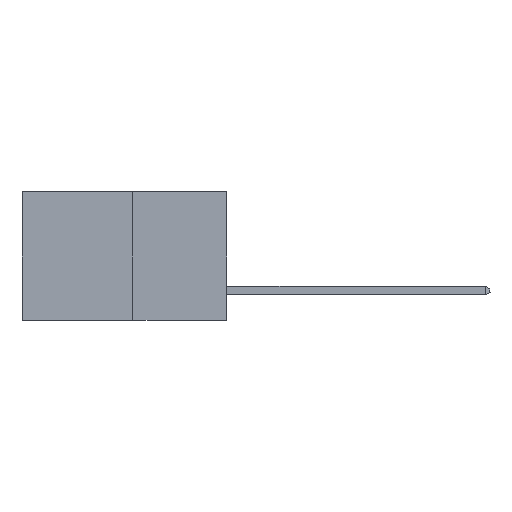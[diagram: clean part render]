
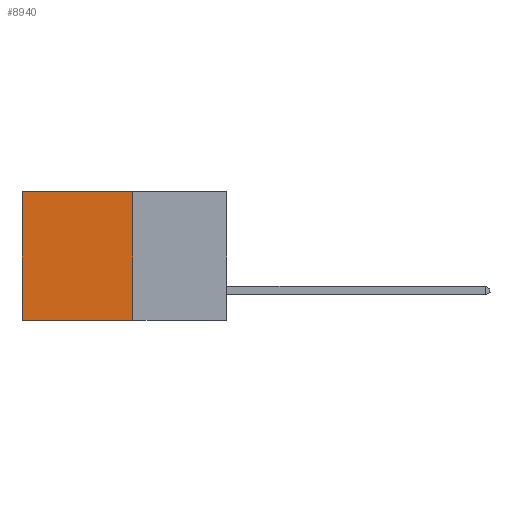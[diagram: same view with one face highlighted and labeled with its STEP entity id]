
A CAD part, left-side view. The second image highlights one B-rep face of the part: STEP entity #8940.
In plain terms, the highlighted planar face has unit normal (-1, 0, 0).
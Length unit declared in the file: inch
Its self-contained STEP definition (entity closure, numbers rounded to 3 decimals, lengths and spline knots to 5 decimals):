
#193 = DIRECTION ( 'NONE',  ( 0., 1., 0. ) ) ;
#296 = CARTESIAN_POINT ( 'NONE',  ( 0.277, 0.27, 0. ) ) ;
#1221 = CARTESIAN_POINT ( 'NONE',  ( 0.277, 0.59, -0.37 ) ) ;
#1253 = EDGE_CURVE ( 'NONE', #1837, #8691, #19390, .T. ) ;
#1837 = VERTEX_POINT ( 'NONE', #17313 ) ;
#3182 = DIRECTION ( 'NONE',  ( 0., 0., -1. ) ) ;
#3802 = ORIENTED_EDGE ( 'NONE', *, *, #19534, .F. ) ;
#5381 = CARTESIAN_POINT ( 'NONE',  ( 0.277, 0.27, -0.37 ) ) ;
#5723 = VECTOR ( 'NONE', #3182, 39.37008 ) ;
#6802 = EDGE_CURVE ( 'NONE', #17176, #8691, #8059, .T. ) ;
#8059 = LINE ( 'NONE', #17835, #20864 ) ;
#8691 = VERTEX_POINT ( 'NONE', #1221 ) ;
#8940 = ADVANCED_FACE ( 'NONE', ( #11349 ), #19799, .F. ) ;
#9045 = DIRECTION ( 'NONE',  ( 0., 0., -1. ) ) ;
#10345 = CARTESIAN_POINT ( 'NONE',  ( 0.277, 0.27, 0. ) ) ;
#10465 = EDGE_CURVE ( 'NONE', #12814, #1837, #13393, .T. ) ;
#10470 = VECTOR ( 'NONE', #9045, 39.37008 ) ;
#11349 = FACE_OUTER_BOUND ( 'NONE', #14837, .T. ) ;
#11478 = ORIENTED_EDGE ( 'NONE', *, *, #1253, .T. ) ;
#11710 = CARTESIAN_POINT ( 'NONE',  ( 0.277, 0.27, -0.37 ) ) ;
#12140 = CARTESIAN_POINT ( 'NONE',  ( 0.277, 0.59, -0.37 ) ) ;
#12814 = VERTEX_POINT ( 'NONE', #10345 ) ;
#12886 = VECTOR ( 'NONE', #193, 39.37008 ) ;
#13393 = LINE ( 'NONE', #296, #12886 ) ;
#14190 = ORIENTED_EDGE ( 'NONE', *, *, #6802, .F. ) ;
#14837 = EDGE_LOOP ( 'NONE', ( #11478, #14190, #3802, #16027 ) ) ;
#15682 = LINE ( 'NONE', #11710, #5723 ) ;
#16027 = ORIENTED_EDGE ( 'NONE', *, *, #10465, .T. ) ;
#17176 = VERTEX_POINT ( 'NONE', #5381 ) ;
#17313 = CARTESIAN_POINT ( 'NONE',  ( 0.277, 0.59, 0. ) ) ;
#17813 = DIRECTION ( 'NONE',  ( 0., 1., 0. ) ) ;
#17835 = CARTESIAN_POINT ( 'NONE',  ( 0.277, 0.27, -0.37 ) ) ;
#19374 = AXIS2_PLACEMENT_3D ( 'NONE', #19778, #19772, #19723 ) ;
#19390 = LINE ( 'NONE', #12140, #10470 ) ;
#19534 = EDGE_CURVE ( 'NONE', #12814, #17176, #15682, .T. ) ;
#19723 = DIRECTION ( 'NONE',  ( 0., 0., -1. ) ) ;
#19772 = DIRECTION ( 'NONE',  ( 1., 0., 0. ) ) ;
#19778 = CARTESIAN_POINT ( 'NONE',  ( 0.277, 0.27, -0.37 ) ) ;
#19799 = PLANE ( 'NONE',  #19374 ) ;
#20864 = VECTOR ( 'NONE', #17813, 39.37008 ) ;
